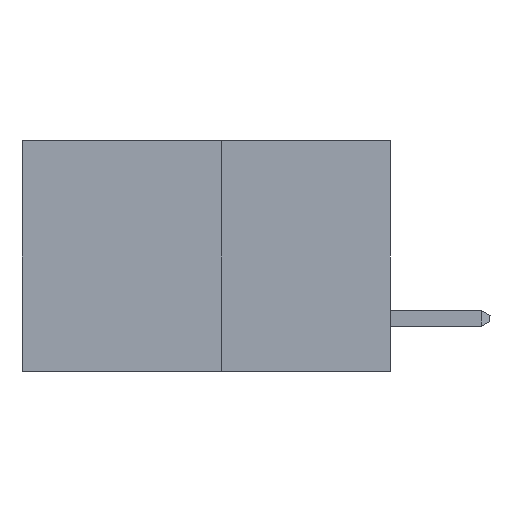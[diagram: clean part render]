
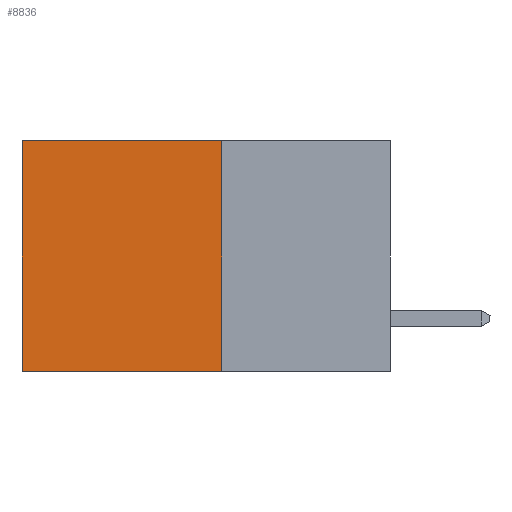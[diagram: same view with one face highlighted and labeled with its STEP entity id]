
A CAD part, left-side view. The second image highlights one B-rep face of the part: STEP entity #8836.
In plain terms, the highlighted planar face has unit normal (-1, 0, 0).
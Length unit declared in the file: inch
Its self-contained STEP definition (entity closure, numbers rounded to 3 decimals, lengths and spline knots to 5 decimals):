
#92 = VERTEX_POINT ( 'NONE', #1128 ) ;
#166 = VERTEX_POINT ( 'NONE', #19144 ) ;
#532 = EDGE_CURVE ( 'NONE', #166, #7672, #10573, .T. ) ;
#1128 = CARTESIAN_POINT ( 'NONE',  ( 0.277, 0.27, 0. ) ) ;
#1547 = LINE ( 'NONE', #5383, #9402 ) ;
#1608 = CARTESIAN_POINT ( 'NONE',  ( 0.277, 0.27, -0.37 ) ) ;
#1732 = EDGE_LOOP ( 'NONE', ( #7532, #5398, #1952, #6608 ) ) ;
#1952 = ORIENTED_EDGE ( 'NONE', *, *, #12668, .F. ) ;
#3683 = DIRECTION ( 'NONE',  ( 0., 0., -1. ) ) ;
#3898 = VECTOR ( 'NONE', #10596, 39.37008 ) ;
#5383 = CARTESIAN_POINT ( 'NONE',  ( 0.277, 0.27, -0.37 ) ) ;
#5398 = ORIENTED_EDGE ( 'NONE', *, *, #10850, .F. ) ;
#5459 = FACE_OUTER_BOUND ( 'NONE', #1732, .T. ) ;
#5613 = DIRECTION ( 'NONE',  ( 0., 0., -1. ) ) ;
#5653 = DIRECTION ( 'NONE',  ( 1., 0., 0. ) ) ;
#5698 = CARTESIAN_POINT ( 'NONE',  ( 0.277, 0.27, -0.37 ) ) ;
#5749 = PLANE ( 'NONE',  #7477 ) ;
#5867 = CARTESIAN_POINT ( 'NONE',  ( 0.277, 0.27, -0.37 ) ) ;
#5944 = CARTESIAN_POINT ( 'NONE',  ( 0.277, 0.27, 0. ) ) ;
#6608 = ORIENTED_EDGE ( 'NONE', *, *, #10654, .T. ) ;
#6953 = DIRECTION ( 'NONE',  ( 0., 0., -1. ) ) ;
#7138 = VERTEX_POINT ( 'NONE', #5867 ) ;
#7274 = CARTESIAN_POINT ( 'NONE',  ( 0.277, 0.59, -0.37 ) ) ;
#7477 = AXIS2_PLACEMENT_3D ( 'NONE', #5698, #5653, #5613 ) ;
#7532 = ORIENTED_EDGE ( 'NONE', *, *, #532, .T. ) ;
#7672 = VERTEX_POINT ( 'NONE', #7274 ) ;
#8043 = LINE ( 'NONE', #5944, #3898 ) ;
#8763 = LINE ( 'NONE', #1608, #16799 ) ;
#8836 = ADVANCED_FACE ( 'NONE', ( #5459 ), #5749, .F. ) ;
#9402 = VECTOR ( 'NONE', #6953, 39.37008 ) ;
#10573 = LINE ( 'NONE', #11723, #15054 ) ;
#10596 = DIRECTION ( 'NONE',  ( 0., 1., 0. ) ) ;
#10654 = EDGE_CURVE ( 'NONE', #92, #166, #8043, .T. ) ;
#10850 = EDGE_CURVE ( 'NONE', #7138, #7672, #8763, .T. ) ;
#10982 = DIRECTION ( 'NONE',  ( 0., 1., 0. ) ) ;
#11723 = CARTESIAN_POINT ( 'NONE',  ( 0.277, 0.59, -0.37 ) ) ;
#12668 = EDGE_CURVE ( 'NONE', #92, #7138, #1547, .T. ) ;
#15054 = VECTOR ( 'NONE', #3683, 39.37008 ) ;
#16799 = VECTOR ( 'NONE', #10982, 39.37008 ) ;
#19144 = CARTESIAN_POINT ( 'NONE',  ( 0.277, 0.59, 0. ) ) ;
